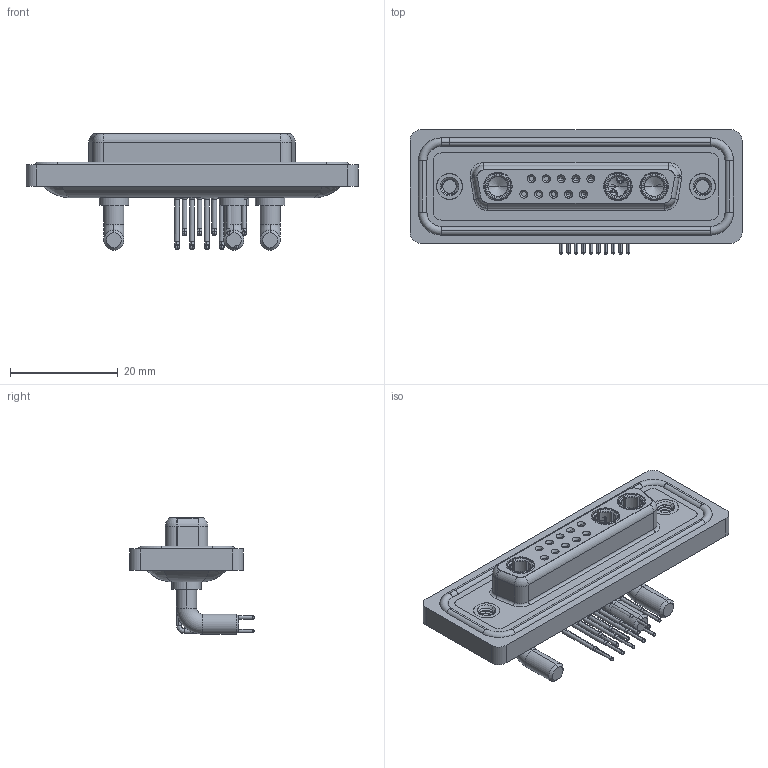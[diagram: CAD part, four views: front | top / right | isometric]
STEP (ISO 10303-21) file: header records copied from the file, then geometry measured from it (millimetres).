
FILE_DESCRIPTION (( 'STEP AP203' ), '1' );
FILE_NAME ('630W13W3240-4NA.STEP', '2024-04-12T01:28:45', ( '' ), ( '' ), 'SwSTEP 2.0', 'SolidWorks 2023', '' );
FILE_SCHEMA (( 'CONFIG_CONTROL_DESIGN' ));
Length unit declared in the file: millimetre
Products named in the file (9): 630Combo Contact Row 1_50 Contacts; 630Combo Contact Row 2_50 Contacts; 630Combo Shell Rear_25 Contacts; 630Combo Waterproof Housing_25 Contacts; 630W13W3240-4NA; Power Socket_40A RA; 630Combo Shell Front_25 Contacts; 630Combo Housing_13W3; 630Combo Threaded Rivet_A
Assembly tree (19 placements, depth 2):
  630W13W3240-4NA
    630Combo Housing_13W3
    630Combo Shell Front_25 Contacts
    630Combo Shell Rear_25 Contacts
    630Combo Threaded Rivet_A  x2
    Power Socket_40A RA  x3
    630Combo Contact Row 1_50 Contacts  x5
    630Combo Contact Row 2_50 Contacts  x5
    630Combo Waterproof Housing_25 Contacts
Bounding box: 61.75 x 23.12 x 21.68 mm (x, y, z)
Volume: 8681.1 mm3; surface area: 14430.8 mm2
Topology: 23 solids, 23 shells, 1144 faces, 2919 edges, 1847 vertices
Faces by surface type: cylinder 491, plane 342, cone 169, torus 89, bspline 53
Entity records: 22655 total; most frequent: CARTESIAN_POINT 5660, DIRECTION 3535, ORIENTED_EDGE 3170, EDGE_CURVE 1585, AXIS2_PLACEMENT_3D 1443, VERTEX_POINT 1013, CIRCLE 789, EDGE_LOOP 746
